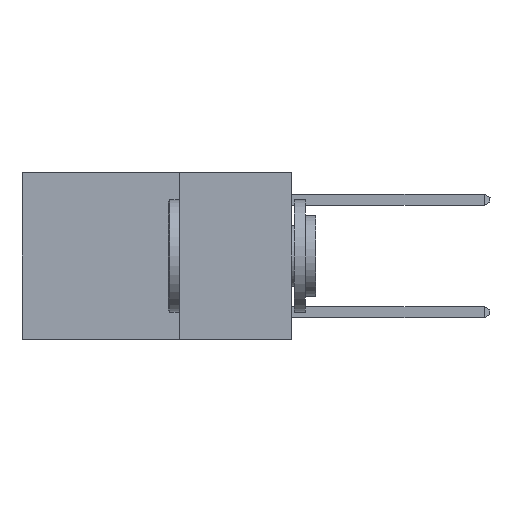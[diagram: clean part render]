
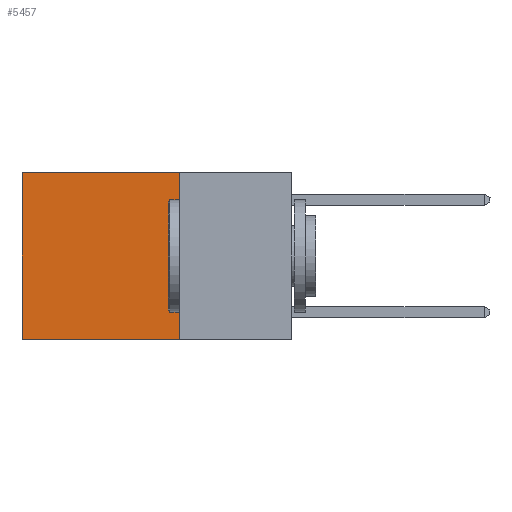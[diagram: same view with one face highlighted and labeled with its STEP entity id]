
A CAD part, left-side view. The second image highlights one B-rep face of the part: STEP entity #5457.
In plain terms, the highlighted planar face has unit normal (-1, 0, 0).
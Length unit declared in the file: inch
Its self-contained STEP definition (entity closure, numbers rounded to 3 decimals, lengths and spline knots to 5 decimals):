
#426 = VERTEX_POINT ( 'NONE', #13497 ) ;
#1082 = CARTESIAN_POINT ( 'NONE',  ( 0.2625, 0.25, 0. ) ) ;
#1435 = CARTESIAN_POINT ( 'NONE',  ( 0.2625, 0.25, -0.37 ) ) ;
#1662 = CARTESIAN_POINT ( 'NONE',  ( 0.2625, 0.25, 0. ) ) ;
#1679 = VECTOR ( 'NONE', #10872, 39.37008 ) ;
#2765 = CARTESIAN_POINT ( 'NONE',  ( 0.2625, 0.6, -0.37 ) ) ;
#2941 = ORIENTED_EDGE ( 'NONE', *, *, #12275, .T. ) ;
#3026 = EDGE_LOOP ( 'NONE', ( #2941, #4514, #5738, #6555 ) ) ;
#3142 = CARTESIAN_POINT ( 'NONE',  ( 0.2625, 0.25, 0. ) ) ;
#3896 = CARTESIAN_POINT ( 'NONE',  ( 0.2625, 0.6, 0. ) ) ;
#4061 = DIRECTION ( 'NONE',  ( 0., 0., -1. ) ) ;
#4208 = VECTOR ( 'NONE', #9220, 39.37008 ) ;
#4514 = ORIENTED_EDGE ( 'NONE', *, *, #13852, .F. ) ;
#4899 = VERTEX_POINT ( 'NONE', #2765 ) ;
#5457 = ADVANCED_FACE ( 'NONE', ( #7360 ), #9841, .F. ) ;
#5738 = ORIENTED_EDGE ( 'NONE', *, *, #11805, .F. ) ;
#5843 = VERTEX_POINT ( 'NONE', #12494 ) ;
#6045 = VECTOR ( 'NONE', #10885, 39.37008 ) ;
#6555 = ORIENTED_EDGE ( 'NONE', *, *, #14996, .T. ) ;
#6625 = DIRECTION ( 'NONE',  ( 0., 0., -1. ) ) ;
#7360 = FACE_OUTER_BOUND ( 'NONE', #3026, .T. ) ;
#9030 = AXIS2_PLACEMENT_3D ( 'NONE', #1662, #11033, #4061 ) ;
#9096 = LINE ( 'NONE', #1435, #6045 ) ;
#9220 = DIRECTION ( 'NONE',  ( 0., 1., 0. ) ) ;
#9841 = PLANE ( 'NONE',  #9030 ) ;
#10291 = VECTOR ( 'NONE', #6625, 39.37008 ) ;
#10377 = LINE ( 'NONE', #1082, #4208 ) ;
#10872 = DIRECTION ( 'NONE',  ( 0., 0., -1. ) ) ;
#10885 = DIRECTION ( 'NONE',  ( 0., 1., 0. ) ) ;
#11033 = DIRECTION ( 'NONE',  ( 1., 0., 0. ) ) ;
#11805 = EDGE_CURVE ( 'NONE', #13384, #426, #12658, .T. ) ;
#12275 = EDGE_CURVE ( 'NONE', #5843, #4899, #13379, .T. ) ;
#12441 = CARTESIAN_POINT ( 'NONE',  ( 0.2625, 0.25, 0. ) ) ;
#12494 = CARTESIAN_POINT ( 'NONE',  ( 0.2625, 0.6, 0. ) ) ;
#12658 = LINE ( 'NONE', #12441, #10291 ) ;
#13379 = LINE ( 'NONE', #3896, #1679 ) ;
#13384 = VERTEX_POINT ( 'NONE', #3142 ) ;
#13497 = CARTESIAN_POINT ( 'NONE',  ( 0.2625, 0.25, -0.37 ) ) ;
#13852 = EDGE_CURVE ( 'NONE', #426, #4899, #9096, .T. ) ;
#14996 = EDGE_CURVE ( 'NONE', #13384, #5843, #10377, .T. ) ;
